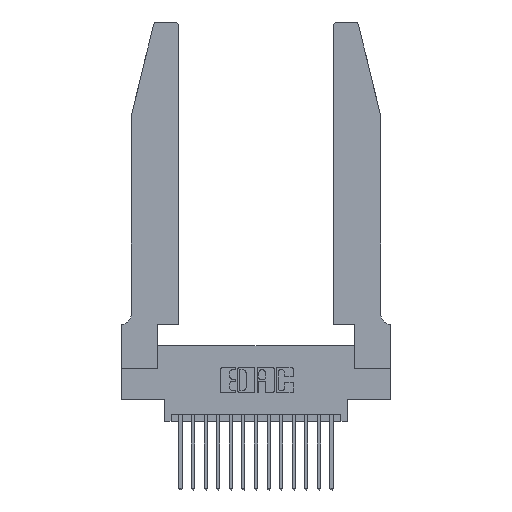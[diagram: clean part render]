
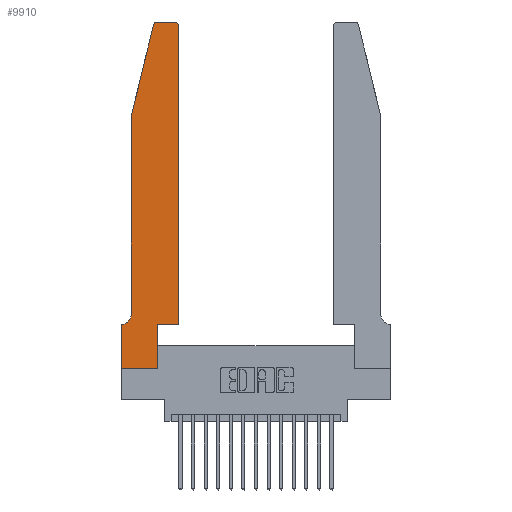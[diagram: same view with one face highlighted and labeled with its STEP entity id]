
A CAD part, top view. The second image highlights one B-rep face of the part: STEP entity #9910.
In plain terms, the highlighted planar face has unit normal (0, 0, 1).
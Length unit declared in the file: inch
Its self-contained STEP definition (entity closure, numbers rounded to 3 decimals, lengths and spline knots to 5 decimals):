
#262 = DIRECTION ( 'NONE',  ( 0., -1., 0. ) ) ;
#312 = DIRECTION ( 'NONE',  ( 1., 0., 0. ) ) ;
#335 = VECTOR ( 'NONE', #262, 39.37008 ) ;
#345 = ORIENTED_EDGE ( 'NONE', *, *, #11180, .T. ) ;
#346 = EDGE_CURVE ( 'NONE', #17946, #14806, #14738, .T. ) ;
#455 = DIRECTION ( 'NONE',  ( 0., 1., 0. ) ) ;
#697 = CARTESIAN_POINT ( 'NONE',  ( 0., 0.35, 0.37 ) ) ;
#699 = CARTESIAN_POINT ( 'NONE',  ( 0.0755, 0.42, 0.37 ) ) ;
#777 = VECTOR ( 'NONE', #455, 39.37008 ) ;
#961 = CARTESIAN_POINT ( 'NONE',  ( 0., 0., 0.37 ) ) ;
#965 = CARTESIAN_POINT ( 'NONE',  ( 0.25487, 2.72718, 0.37 ) ) ;
#1303 = ORIENTED_EDGE ( 'NONE', *, *, #13443, .T. ) ;
#1393 = CARTESIAN_POINT ( 'NONE',  ( 0.4505, 0.35, 0.37 ) ) ;
#1435 = AXIS2_PLACEMENT_3D ( 'NONE', #6299, #16424, #312 ) ;
#1511 = ORIENTED_EDGE ( 'NONE', *, *, #346, .T. ) ;
#1551 = CIRCLE ( 'NONE', #1435, 0.03 ) ;
#1810 = LINE ( 'NONE', #8711, #12824 ) ;
#1834 = VECTOR ( 'NONE', #6743, 39.37008 ) ;
#2543 = EDGE_CURVE ( 'NONE', #7904, #17946, #1810, .T. ) ;
#2646 = LINE ( 'NONE', #3123, #335 ) ;
#2779 = FACE_OUTER_BOUND ( 'NONE', #11819, .T. ) ;
#2952 = CARTESIAN_POINT ( 'NONE',  ( 0.0755, 0.35, 0.37 ) ) ;
#2988 = CARTESIAN_POINT ( 'NONE',  ( 0.2865, 0.35, 0.37 ) ) ;
#3099 = EDGE_CURVE ( 'NONE', #12883, #7120, #17442, .T. ) ;
#3123 = CARTESIAN_POINT ( 'NONE',  ( 0.0755, 2., 0.37 ) ) ;
#3252 = DIRECTION ( 'NONE',  ( 0., 0., -1. ) ) ;
#3457 = CARTESIAN_POINT ( 'NONE',  ( 0.0755, 2., 0.37 ) ) ;
#3495 = AXIS2_PLACEMENT_3D ( 'NONE', #697, #17048, #16872 ) ;
#3624 = CARTESIAN_POINT ( 'NONE',  ( 0.4505, 0.35, 0.37 ) ) ;
#3725 = AXIS2_PLACEMENT_3D ( 'NONE', #14696, #17716, #14637 ) ;
#4054 = EDGE_CURVE ( 'NONE', #8693, #18255, #1551, .T. ) ;
#4063 = LINE ( 'NONE', #3624, #18292 ) ;
#4677 = CARTESIAN_POINT ( 'NONE',  ( 0.2605, 2.75, 0.37 ) ) ;
#5797 = EDGE_CURVE ( 'NONE', #15199, #14786, #4063, .T. ) ;
#6299 = CARTESIAN_POINT ( 'NONE',  ( 0.4205, 2.72, 0.37 ) ) ;
#6437 = LINE ( 'NONE', #2952, #10108 ) ;
#6486 = DIRECTION ( 'NONE',  ( 1., 0., 0. ) ) ;
#6586 = LINE ( 'NONE', #1393, #17833 ) ;
#6743 = DIRECTION ( 'NONE',  ( -0.239, -0.971, 0. ) ) ;
#6791 = PLANE ( 'NONE',  #3495 ) ;
#6798 = CARTESIAN_POINT ( 'NONE',  ( 0.4505, 0.35, 0.37 ) ) ;
#7120 = VERTEX_POINT ( 'NONE', #14460 ) ;
#7197 = EDGE_CURVE ( 'NONE', #7120, #15721, #2646, .T. ) ;
#7904 = VERTEX_POINT ( 'NONE', #9124 ) ;
#8071 = ORIENTED_EDGE ( 'NONE', *, *, #5797, .T. ) ;
#8163 = ORIENTED_EDGE ( 'NONE', *, *, #16793, .T. ) ;
#8178 = CARTESIAN_POINT ( 'NONE',  ( 0.4505, 2.72, 0.37 ) ) ;
#8233 = VECTOR ( 'NONE', #13893, 39.37008 ) ;
#8693 = VERTEX_POINT ( 'NONE', #8178 ) ;
#8711 = CARTESIAN_POINT ( 'NONE',  ( 0., 0., 0.37 ) ) ;
#9124 = CARTESIAN_POINT ( 'NONE',  ( 0., 0.35, 0.37 ) ) ;
#9691 = CARTESIAN_POINT ( 'NONE',  ( 0.2865, 0., 0.37 ) ) ;
#9910 = ADVANCED_FACE ( 'NONE', ( #2779 ), #6791, .T. ) ;
#9967 = ORIENTED_EDGE ( 'NONE', *, *, #12473, .T. ) ;
#10108 = VECTOR ( 'NONE', #13192, 39.37008 ) ;
#10753 = ORIENTED_EDGE ( 'NONE', *, *, #4054, .T. ) ;
#11180 = EDGE_CURVE ( 'NONE', #18255, #12304, #15556, .T. ) ;
#11819 = EDGE_LOOP ( 'NONE', ( #345, #18922, #16477, #13940, #1303, #9967, #16554, #1511, #8163, #8071, #14124, #10753 ) ) ;
#12034 = CARTESIAN_POINT ( 'NONE',  ( 0.0055, 0.42, 0.37 ) ) ;
#12304 = VERTEX_POINT ( 'NONE', #13802 ) ;
#12473 = EDGE_CURVE ( 'NONE', #15887, #7904, #6437, .T. ) ;
#12824 = VECTOR ( 'NONE', #13122, 39.37008 ) ;
#12883 = VERTEX_POINT ( 'NONE', #965 ) ;
#13122 = DIRECTION ( 'NONE',  ( 0., -1., 0. ) ) ;
#13192 = DIRECTION ( 'NONE',  ( -1., 0., 0. ) ) ;
#13443 = EDGE_CURVE ( 'NONE', #15721, #15887, #18608, .T. ) ;
#13802 = CARTESIAN_POINT ( 'NONE',  ( 0.284, 2.75, 0.37 ) ) ;
#13893 = DIRECTION ( 'NONE',  ( -1., 0., 0. ) ) ;
#13940 = ORIENTED_EDGE ( 'NONE', *, *, #7197, .T. ) ;
#14124 = ORIENTED_EDGE ( 'NONE', *, *, #15933, .T. ) ;
#14460 = CARTESIAN_POINT ( 'NONE',  ( 0.0755, 2., 0.37 ) ) ;
#14637 = DIRECTION ( 'NONE',  ( 1., 0., 0. ) ) ;
#14679 = DIRECTION ( 'NONE',  ( 0., 1., 0. ) ) ;
#14696 = CARTESIAN_POINT ( 'NONE',  ( 0.284, 2.72, 0.37 ) ) ;
#14738 = LINE ( 'NONE', #961, #16109 ) ;
#14786 = VERTEX_POINT ( 'NONE', #6798 ) ;
#14796 = LINE ( 'NONE', #16700, #777 ) ;
#14806 = VERTEX_POINT ( 'NONE', #9691 ) ;
#15199 = VERTEX_POINT ( 'NONE', #2988 ) ;
#15556 = LINE ( 'NONE', #4677, #8233 ) ;
#15721 = VERTEX_POINT ( 'NONE', #699 ) ;
#15780 = DIRECTION ( 'NONE',  ( 1., 0., 0. ) ) ;
#15887 = VERTEX_POINT ( 'NONE', #17570 ) ;
#15933 = EDGE_CURVE ( 'NONE', #14786, #8693, #6586, .T. ) ;
#16109 = VECTOR ( 'NONE', #15780, 39.37008 ) ;
#16424 = DIRECTION ( 'NONE',  ( 0., 0., 1. ) ) ;
#16466 = CARTESIAN_POINT ( 'NONE',  ( 0., 0., 0.37 ) ) ;
#16477 = ORIENTED_EDGE ( 'NONE', *, *, #3099, .T. ) ;
#16540 = AXIS2_PLACEMENT_3D ( 'NONE', #12034, #3252, #17990 ) ;
#16554 = ORIENTED_EDGE ( 'NONE', *, *, #2543, .T. ) ;
#16700 = CARTESIAN_POINT ( 'NONE',  ( 0.2865, 0.35, 0.37 ) ) ;
#16793 = EDGE_CURVE ( 'NONE', #14806, #15199, #14796, .T. ) ;
#16872 = DIRECTION ( 'NONE',  ( 1., 0., 0. ) ) ;
#17048 = DIRECTION ( 'NONE',  ( 0., 0., 1. ) ) ;
#17442 = LINE ( 'NONE', #3457, #1834 ) ;
#17570 = CARTESIAN_POINT ( 'NONE',  ( 0.0055, 0.35, 0.37 ) ) ;
#17716 = DIRECTION ( 'NONE',  ( 0., 0., 1. ) ) ;
#17833 = VECTOR ( 'NONE', #14679, 39.37008 ) ;
#17946 = VERTEX_POINT ( 'NONE', #16466 ) ;
#17990 = DIRECTION ( 'NONE',  ( -1., 0., 0. ) ) ;
#18255 = VERTEX_POINT ( 'NONE', #18957 ) ;
#18292 = VECTOR ( 'NONE', #6486, 39.37008 ) ;
#18608 = CIRCLE ( 'NONE', #16540, 0.07 ) ;
#18883 = CIRCLE ( 'NONE', #3725, 0.03 ) ;
#18895 = EDGE_CURVE ( 'NONE', #12304, #12883, #18883, .T. ) ;
#18922 = ORIENTED_EDGE ( 'NONE', *, *, #18895, .T. ) ;
#18957 = CARTESIAN_POINT ( 'NONE',  ( 0.4205, 2.75, 0.37 ) ) ;
